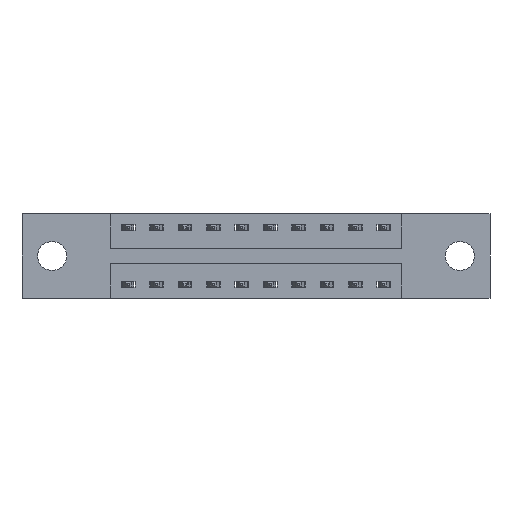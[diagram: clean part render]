
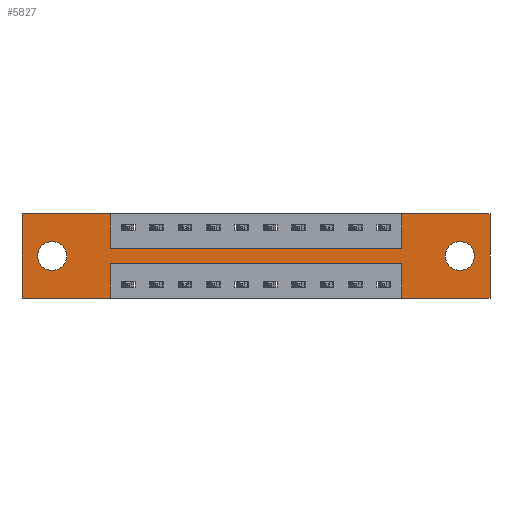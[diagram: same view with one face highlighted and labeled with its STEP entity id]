
A CAD part, front view. The second image highlights one B-rep face of the part: STEP entity #5827.
In plain terms, the highlighted planar face has unit normal (0, -1, 0).
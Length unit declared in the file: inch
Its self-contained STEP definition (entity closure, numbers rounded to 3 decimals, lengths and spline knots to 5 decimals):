
#13 = DIRECTION ( 'NONE',  ( 0., 0., -1. ) ) ;
#44 = DIRECTION ( 'NONE',  ( -1., 0., 0. ) ) ;
#64 = ORIENTED_EDGE ( 'NONE', *, *, #6628, .F. ) ;
#260 = VECTOR ( 'NONE', #6997, 39.37008 ) ;
#330 = LINE ( 'NONE', #7211, #2321 ) ;
#357 = DIRECTION ( 'NONE',  ( 0., 0., -1. ) ) ;
#373 = EDGE_CURVE ( 'NONE', #7131, #999, #3739, .T. ) ;
#389 = VECTOR ( 'NONE', #5558, 39.37008 ) ;
#430 = ORIENTED_EDGE ( 'NONE', *, *, #3064, .T. ) ;
#455 = EDGE_CURVE ( 'NONE', #6772, #9388, #5775, .T. ) ;
#585 = DIRECTION ( 'NONE',  ( 0., 1., 0. ) ) ;
#639 = LINE ( 'NONE', #3165, #1421 ) ;
#720 = LINE ( 'NONE', #8208, #3882 ) ;
#861 = CARTESIAN_POINT ( 'NONE',  ( 0., 0., -0.37 ) ) ;
#889 = CARTESIAN_POINT ( 'NONE',  ( 1.9275, 0., -0.121 ) ) ;
#963 = ORIENTED_EDGE ( 'NONE', *, *, #5893, .F. ) ;
#999 = VERTEX_POINT ( 'NONE', #8302 ) ;
#1183 = LINE ( 'NONE', #7897, #3402 ) ;
#1210 = ORIENTED_EDGE ( 'NONE', *, *, #9738, .T. ) ;
#1421 = VECTOR ( 'NONE', #9118, 39.37008 ) ;
#1442 = AXIS2_PLACEMENT_3D ( 'NONE', #9642, #6358, #9709 ) ;
#1446 = CARTESIAN_POINT ( 'NONE',  ( 0.3875, 0., -0.37 ) ) ;
#1499 = EDGE_CURVE ( 'NONE', #8013, #6226, #3595, .T. ) ;
#1698 = ORIENTED_EDGE ( 'NONE', *, *, #4252, .F. ) ;
#1809 = CARTESIAN_POINT ( 'NONE',  ( 0.1325, 0., -0.121 ) ) ;
#1835 = VECTOR ( 'NONE', #8042, 39.37008 ) ;
#1908 = ORIENTED_EDGE ( 'NONE', *, *, #4607, .F. ) ;
#1911 = ORIENTED_EDGE ( 'NONE', *, *, #3059, .F. ) ;
#2112 = VECTOR ( 'NONE', #10022, 39.37008 ) ;
#2206 = CARTESIAN_POINT ( 'NONE',  ( 0., 0., -0.37 ) ) ;
#2257 = FACE_BOUND ( 'NONE', #8874, .T. ) ;
#2291 = VECTOR ( 'NONE', #3904, 39.37008 ) ;
#2321 = VECTOR ( 'NONE', #10546, 39.37008 ) ;
#2354 = CARTESIAN_POINT ( 'NONE',  ( 0., 0., 0. ) ) ;
#2374 = CARTESIAN_POINT ( 'NONE',  ( 0., 0., 0. ) ) ;
#2498 = CIRCLE ( 'NONE', #1442, 0.064 ) ;
#2616 = VECTOR ( 'NONE', #5905, 39.37008 ) ;
#2830 = ORIENTED_EDGE ( 'NONE', *, *, #1499, .F. ) ;
#2848 = CARTESIAN_POINT ( 'NONE',  ( 1.6725, 0., -0.37 ) ) ;
#3059 = EDGE_CURVE ( 'NONE', #7456, #7131, #1183, .T. ) ;
#3064 = EDGE_CURVE ( 'NONE', #3680, #4243, #2498, .T. ) ;
#3156 = VERTEX_POINT ( 'NONE', #4085 ) ;
#3165 = CARTESIAN_POINT ( 'NONE',  ( 0.3875, 0., -0.22 ) ) ;
#3299 = ORIENTED_EDGE ( 'NONE', *, *, #10004, .T. ) ;
#3306 = CARTESIAN_POINT ( 'NONE',  ( 0.3875, 0., -0.37 ) ) ;
#3338 = DIRECTION ( 'NONE',  ( 0., -1., 0. ) ) ;
#3402 = VECTOR ( 'NONE', #357, 39.37008 ) ;
#3416 = DIRECTION ( 'NONE',  ( 0., 1., 0. ) ) ;
#3595 = LINE ( 'NONE', #5156, #6894 ) ;
#3680 = VERTEX_POINT ( 'NONE', #1809 ) ;
#3739 = LINE ( 'NONE', #4689, #1835 ) ;
#3812 = ORIENTED_EDGE ( 'NONE', *, *, #10821, .F. ) ;
#3814 = DIRECTION ( 'NONE',  ( 0., 1., 0. ) ) ;
#3882 = VECTOR ( 'NONE', #7557, 39.37008 ) ;
#3904 = DIRECTION ( 'NONE',  ( -1., 0., 0. ) ) ;
#3935 = EDGE_CURVE ( 'NONE', #9388, #9587, #8238, .T. ) ;
#4021 = CARTESIAN_POINT ( 'NONE',  ( 1.6725, 0., -0.22 ) ) ;
#4070 = VERTEX_POINT ( 'NONE', #5324 ) ;
#4085 = CARTESIAN_POINT ( 'NONE',  ( 1.6725, 0., -0.37 ) ) ;
#4243 = VERTEX_POINT ( 'NONE', #7054 ) ;
#4252 = EDGE_CURVE ( 'NONE', #3156, #6641, #10232, .T. ) ;
#4280 = ORIENTED_EDGE ( 'NONE', *, *, #6690, .F. ) ;
#4607 = EDGE_CURVE ( 'NONE', #6641, #5447, #639, .T. ) ;
#4689 = CARTESIAN_POINT ( 'NONE',  ( 0.3875, 0., -0.15 ) ) ;
#5024 = DIRECTION ( 'NONE',  ( 0., 0., -1. ) ) ;
#5057 = CARTESIAN_POINT ( 'NONE',  ( 0., 0., -0.37 ) ) ;
#5156 = CARTESIAN_POINT ( 'NONE',  ( 2.06, 0., 0. ) ) ;
#5323 = AXIS2_PLACEMENT_3D ( 'NONE', #8228, #585, #8082 ) ;
#5324 = CARTESIAN_POINT ( 'NONE',  ( 1.9275, 0., -0.249 ) ) ;
#5378 = DIRECTION ( 'NONE',  ( 0., 0., -1. ) ) ;
#5447 = VERTEX_POINT ( 'NONE', #5685 ) ;
#5558 = DIRECTION ( 'NONE',  ( 0., 0., 1. ) ) ;
#5615 = FACE_BOUND ( 'NONE', #10059, .T. ) ;
#5685 = CARTESIAN_POINT ( 'NONE',  ( 0.3875, 0., -0.22 ) ) ;
#5686 = LINE ( 'NONE', #2374, #2112 ) ;
#5775 = LINE ( 'NONE', #861, #5897 ) ;
#5815 = DIRECTION ( 'NONE',  ( 0., 0., -1. ) ) ;
#5827 = ADVANCED_FACE ( 'NONE', ( #2257, #5615, #9752 ), #9170, .T. ) ;
#5845 = CIRCLE ( 'NONE', #5323, 0.064 ) ;
#5893 = EDGE_CURVE ( 'NONE', #6226, #3156, #7532, .T. ) ;
#5897 = VECTOR ( 'NONE', #44, 39.37008 ) ;
#5905 = DIRECTION ( 'NONE',  ( 0., 0., -1. ) ) ;
#6157 = AXIS2_PLACEMENT_3D ( 'NONE', #8422, #3416, #5024 ) ;
#6217 = CIRCLE ( 'NONE', #9183, 0.064 ) ;
#6226 = VERTEX_POINT ( 'NONE', #6423 ) ;
#6358 = DIRECTION ( 'NONE',  ( 0., 1., 0. ) ) ;
#6423 = CARTESIAN_POINT ( 'NONE',  ( 2.06, 0., -0.37 ) ) ;
#6498 = ORIENTED_EDGE ( 'NONE', *, *, #455, .F. ) ;
#6628 = EDGE_CURVE ( 'NONE', #999, #6966, #720, .T. ) ;
#6641 = VERTEX_POINT ( 'NONE', #4021 ) ;
#6690 = EDGE_CURVE ( 'NONE', #9587, #7456, #5686, .T. ) ;
#6701 = AXIS2_PLACEMENT_3D ( 'NONE', #5057, #3338, #5815 ) ;
#6772 = VERTEX_POINT ( 'NONE', #1446 ) ;
#6894 = VECTOR ( 'NONE', #13, 39.37008 ) ;
#6966 = VERTEX_POINT ( 'NONE', #9535 ) ;
#6997 = DIRECTION ( 'NONE',  ( 0., 0., 1. ) ) ;
#7018 = ORIENTED_EDGE ( 'NONE', *, *, #10816, .T. ) ;
#7054 = CARTESIAN_POINT ( 'NONE',  ( 0.1325, 0., -0.249 ) ) ;
#7131 = VERTEX_POINT ( 'NONE', #8318 ) ;
#7211 = CARTESIAN_POINT ( 'NONE',  ( 0., 0., 0. ) ) ;
#7383 = CIRCLE ( 'NONE', #6157, 0.064 ) ;
#7456 = VERTEX_POINT ( 'NONE', #7873 ) ;
#7471 = EDGE_CURVE ( 'NONE', #6966, #8013, #330, .T. ) ;
#7532 = LINE ( 'NONE', #8096, #2291 ) ;
#7557 = DIRECTION ( 'NONE',  ( 0., 0., 1. ) ) ;
#7716 = CARTESIAN_POINT ( 'NONE',  ( 0., 0., 0. ) ) ;
#7837 = ORIENTED_EDGE ( 'NONE', *, *, #3935, .F. ) ;
#7873 = CARTESIAN_POINT ( 'NONE',  ( 0.3875, 0., 0. ) ) ;
#7897 = CARTESIAN_POINT ( 'NONE',  ( 0.3875, 0., 0. ) ) ;
#8013 = VERTEX_POINT ( 'NONE', #10025 ) ;
#8042 = DIRECTION ( 'NONE',  ( 1., 0., 0. ) ) ;
#8082 = DIRECTION ( 'NONE',  ( 0., 0., 1. ) ) ;
#8096 = CARTESIAN_POINT ( 'NONE',  ( 0., 0., -0.37 ) ) ;
#8208 = CARTESIAN_POINT ( 'NONE',  ( 1.6725, 0., 0. ) ) ;
#8228 = CARTESIAN_POINT ( 'NONE',  ( 0.1325, 0., -0.185 ) ) ;
#8238 = LINE ( 'NONE', #2354, #389 ) ;
#8302 = CARTESIAN_POINT ( 'NONE',  ( 1.6725, 0., -0.15 ) ) ;
#8318 = CARTESIAN_POINT ( 'NONE',  ( 0.3875, 0., -0.15 ) ) ;
#8422 = CARTESIAN_POINT ( 'NONE',  ( 1.9275, 0., -0.185 ) ) ;
#8874 = EDGE_LOOP ( 'NONE', ( #7018, #3299 ) ) ;
#8918 = EDGE_LOOP ( 'NONE', ( #3812, #1908, #1698, #963, #2830, #8979, #64, #10123, #1911, #4280, #7837, #6498 ) ) ;
#8979 = ORIENTED_EDGE ( 'NONE', *, *, #7471, .F. ) ;
#9092 = VERTEX_POINT ( 'NONE', #889 ) ;
#9118 = DIRECTION ( 'NONE',  ( -1., 0., 0. ) ) ;
#9139 = LINE ( 'NONE', #3306, #2616 ) ;
#9170 = PLANE ( 'NONE',  #6701 ) ;
#9183 = AXIS2_PLACEMENT_3D ( 'NONE', #10526, #3814, #5378 ) ;
#9388 = VERTEX_POINT ( 'NONE', #2206 ) ;
#9535 = CARTESIAN_POINT ( 'NONE',  ( 1.6725, 0., 0. ) ) ;
#9587 = VERTEX_POINT ( 'NONE', #7716 ) ;
#9642 = CARTESIAN_POINT ( 'NONE',  ( 0.1325, 0., -0.185 ) ) ;
#9709 = DIRECTION ( 'NONE',  ( 0., 0., 1. ) ) ;
#9738 = EDGE_CURVE ( 'NONE', #4243, #3680, #5845, .T. ) ;
#9752 = FACE_OUTER_BOUND ( 'NONE', #8918, .T. ) ;
#10004 = EDGE_CURVE ( 'NONE', #4070, #9092, #6217, .T. ) ;
#10022 = DIRECTION ( 'NONE',  ( 1., 0., 0. ) ) ;
#10025 = CARTESIAN_POINT ( 'NONE',  ( 2.06, 0., 0. ) ) ;
#10059 = EDGE_LOOP ( 'NONE', ( #430, #1210 ) ) ;
#10123 = ORIENTED_EDGE ( 'NONE', *, *, #373, .F. ) ;
#10232 = LINE ( 'NONE', #2848, #260 ) ;
#10526 = CARTESIAN_POINT ( 'NONE',  ( 1.9275, 0., -0.185 ) ) ;
#10546 = DIRECTION ( 'NONE',  ( 1., 0., 0. ) ) ;
#10816 = EDGE_CURVE ( 'NONE', #9092, #4070, #7383, .T. ) ;
#10821 = EDGE_CURVE ( 'NONE', #5447, #6772, #9139, .T. ) ;
